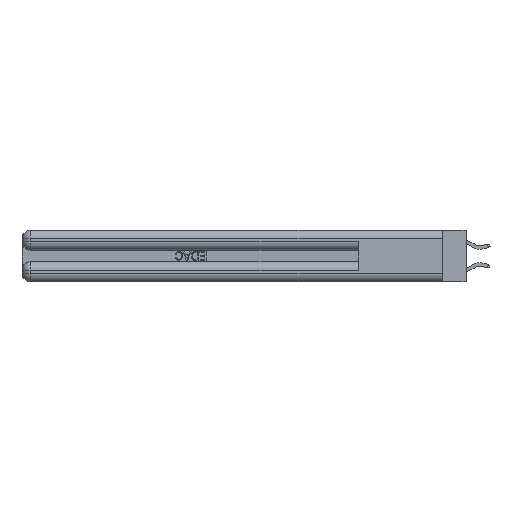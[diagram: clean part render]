
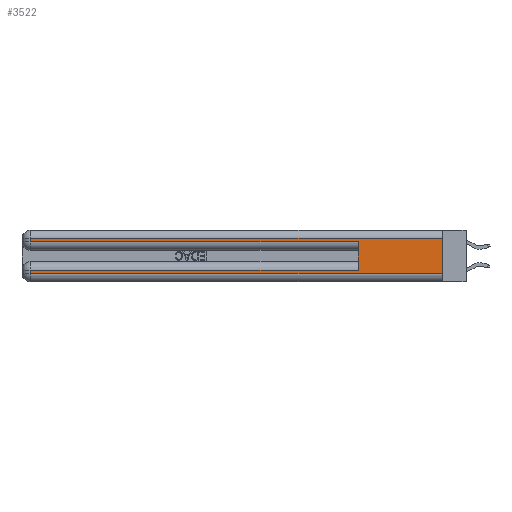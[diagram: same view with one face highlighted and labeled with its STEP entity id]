
A CAD part, left-side view. The second image highlights one B-rep face of the part: STEP entity #3522.
In plain terms, the highlighted planar face has unit normal (-1, 0, 0).
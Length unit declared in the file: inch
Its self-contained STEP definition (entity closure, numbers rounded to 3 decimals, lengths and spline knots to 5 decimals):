
#285 = VECTOR ( 'NONE', #26127, 39.37008 ) ;
#333 = VERTEX_POINT ( 'NONE', #2430 ) ;
#723 = VERTEX_POINT ( 'NONE', #15733 ) ;
#739 = LINE ( 'NONE', #13278, #1180 ) ;
#1180 = VECTOR ( 'NONE', #18633, 39.37008 ) ;
#1354 = CARTESIAN_POINT ( 'NONE',  ( 0., 2.94, 0.37 ) ) ;
#1754 = VERTEX_POINT ( 'NONE', #4680 ) ;
#2321 = VECTOR ( 'NONE', #13736, 39.37008 ) ;
#2430 = CARTESIAN_POINT ( 'NONE',  ( 0., 0.6, 0.285 ) ) ;
#2587 = CARTESIAN_POINT ( 'NONE',  ( 0., 0., 0.285 ) ) ;
#3522 = ADVANCED_FACE ( 'NONE', ( #25294 ), #30108, .F. ) ;
#4628 = VERTEX_POINT ( 'NONE', #18862 ) ;
#4653 = LINE ( 'NONE', #12150, #12694 ) ;
#4680 = CARTESIAN_POINT ( 'NONE',  ( 0., 0., 0.31 ) ) ;
#5036 = ORIENTED_EDGE ( 'NONE', *, *, #31614, .T. ) ;
#5802 = EDGE_CURVE ( 'NONE', #16817, #723, #32661, .T. ) ;
#7926 = VECTOR ( 'NONE', #20069, 39.37008 ) ;
#8893 = DIRECTION ( 'NONE',  ( 0., 0., -1. ) ) ;
#9893 = CARTESIAN_POINT ( 'NONE',  ( 0., 0., 0.085 ) ) ;
#10379 = EDGE_CURVE ( 'NONE', #1754, #10490, #11282, .T. ) ;
#10490 = VERTEX_POINT ( 'NONE', #31401 ) ;
#10663 = ORIENTED_EDGE ( 'NONE', *, *, #5802, .T. ) ;
#11282 = LINE ( 'NONE', #26448, #285 ) ;
#11993 = ORIENTED_EDGE ( 'NONE', *, *, #18757, .T. ) ;
#12150 = CARTESIAN_POINT ( 'NONE',  ( 0., 0., 0.06 ) ) ;
#12632 = DIRECTION ( 'NONE',  ( 1., 0., 0. ) ) ;
#12694 = VECTOR ( 'NONE', #30110, 39.37008 ) ;
#13278 = CARTESIAN_POINT ( 'NONE',  ( 0., 0.6, 0.145 ) ) ;
#13336 = CARTESIAN_POINT ( 'NONE',  ( 0., 0.6, 0.085 ) ) ;
#13714 = EDGE_CURVE ( 'NONE', #4628, #16606, #4653, .T. ) ;
#13736 = DIRECTION ( 'NONE',  ( 0., 0., -1. ) ) ;
#14019 = EDGE_LOOP ( 'NONE', ( #21468, #19375, #5036, #11993, #15184, #10663, #30277, #22592 ) ) ;
#14547 = LINE ( 'NONE', #1354, #32053 ) ;
#15184 = ORIENTED_EDGE ( 'NONE', *, *, #21680, .F. ) ;
#15733 = CARTESIAN_POINT ( 'NONE',  ( 0., 2.94, 0.085 ) ) ;
#16536 = CARTESIAN_POINT ( 'NONE',  ( 0., 0., 0.06 ) ) ;
#16606 = VERTEX_POINT ( 'NONE', #16536 ) ;
#16817 = VERTEX_POINT ( 'NONE', #13336 ) ;
#16874 = CARTESIAN_POINT ( 'NONE',  ( 0., 0., 0.37 ) ) ;
#17208 = LINE ( 'NONE', #16874, #32095 ) ;
#18633 = DIRECTION ( 'NONE',  ( 0., 0., 1. ) ) ;
#18757 = EDGE_CURVE ( 'NONE', #28633, #333, #29917, .T. ) ;
#18862 = CARTESIAN_POINT ( 'NONE',  ( 0., 2.94, 0.06 ) ) ;
#19375 = ORIENTED_EDGE ( 'NONE', *, *, #10379, .T. ) ;
#20069 = DIRECTION ( 'NONE',  ( 0., 1., 0. ) ) ;
#21468 = ORIENTED_EDGE ( 'NONE', *, *, #31393, .F. ) ;
#21680 = EDGE_CURVE ( 'NONE', #16817, #333, #739, .T. ) ;
#22364 = EDGE_CURVE ( 'NONE', #723, #4628, #14547, .T. ) ;
#22592 = ORIENTED_EDGE ( 'NONE', *, *, #13714, .T. ) ;
#22783 = DIRECTION ( 'NONE',  ( 0., 0., -1. ) ) ;
#23218 = LINE ( 'NONE', #23556, #2321 ) ;
#23556 = CARTESIAN_POINT ( 'NONE',  ( 0., 2.94, 0.37 ) ) ;
#24494 = CARTESIAN_POINT ( 'NONE',  ( 0., 2.94, 0.285 ) ) ;
#24944 = DIRECTION ( 'NONE',  ( 0., -1., 0. ) ) ;
#25294 = FACE_OUTER_BOUND ( 'NONE', #14019, .T. ) ;
#25646 = CARTESIAN_POINT ( 'NONE',  ( 0., 0., 0.37 ) ) ;
#26127 = DIRECTION ( 'NONE',  ( 0., 1., 0. ) ) ;
#26448 = CARTESIAN_POINT ( 'NONE',  ( 0., 0., 0.31 ) ) ;
#27021 = DIRECTION ( 'NONE',  ( 0., 0., -1. ) ) ;
#28197 = AXIS2_PLACEMENT_3D ( 'NONE', #25646, #12632, #22783 ) ;
#28211 = VECTOR ( 'NONE', #24944, 39.37008 ) ;
#28633 = VERTEX_POINT ( 'NONE', #24494 ) ;
#29917 = LINE ( 'NONE', #2587, #28211 ) ;
#30108 = PLANE ( 'NONE',  #28197 ) ;
#30110 = DIRECTION ( 'NONE',  ( 0., -1., 0. ) ) ;
#30277 = ORIENTED_EDGE ( 'NONE', *, *, #22364, .T. ) ;
#31393 = EDGE_CURVE ( 'NONE', #1754, #16606, #17208, .T. ) ;
#31401 = CARTESIAN_POINT ( 'NONE',  ( 0., 2.94, 0.31 ) ) ;
#31614 = EDGE_CURVE ( 'NONE', #10490, #28633, #23218, .T. ) ;
#32053 = VECTOR ( 'NONE', #8893, 39.37008 ) ;
#32095 = VECTOR ( 'NONE', #27021, 39.37008 ) ;
#32661 = LINE ( 'NONE', #9893, #7926 ) ;
